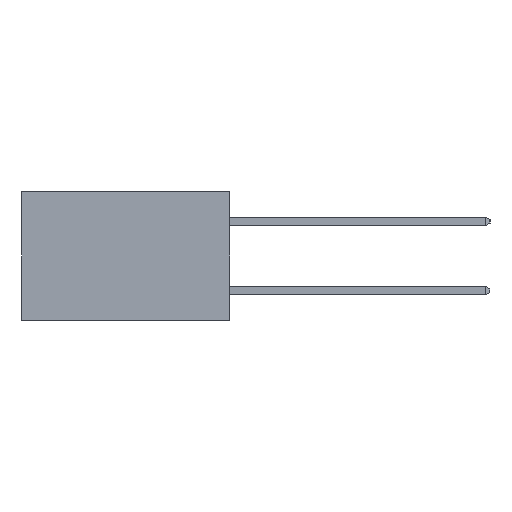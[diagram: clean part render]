
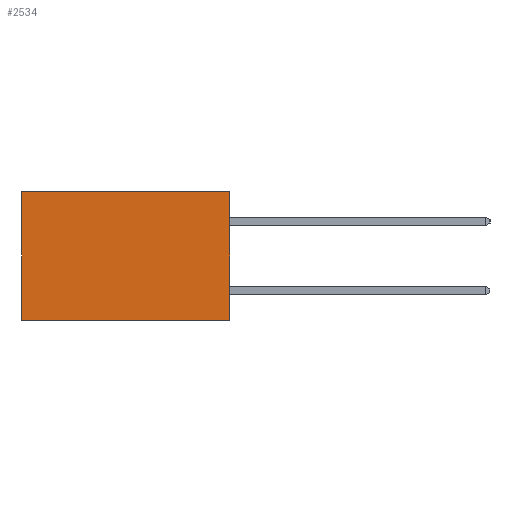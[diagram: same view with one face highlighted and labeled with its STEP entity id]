
A CAD part, left-side view. The second image highlights one B-rep face of the part: STEP entity #2534.
In plain terms, the highlighted planar face has unit normal (-1, 0, 0).
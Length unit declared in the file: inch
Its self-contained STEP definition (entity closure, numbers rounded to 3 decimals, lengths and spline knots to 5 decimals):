
#65 = DIRECTION ( 'NONE',  ( 1., 0., 0. ) ) ;
#964 = LINE ( 'NONE', #3875, #15997 ) ;
#1285 = CARTESIAN_POINT ( 'NONE',  ( 0.298, 0., 0. ) ) ;
#1980 = EDGE_CURVE ( 'NONE', #6765, #12540, #15928, .T. ) ;
#2534 = ADVANCED_FACE ( 'NONE', ( #10368 ), #13266, .F. ) ;
#2613 = VECTOR ( 'NONE', #5511, 39.37008 ) ;
#2827 = DIRECTION ( 'NONE',  ( 0., 1., 0. ) ) ;
#3875 = CARTESIAN_POINT ( 'NONE',  ( 0.298, 0.6, 0. ) ) ;
#4779 = EDGE_CURVE ( 'NONE', #13576, #14364, #964, .T. ) ;
#5061 = CARTESIAN_POINT ( 'NONE',  ( 0.298, 0., -0.37 ) ) ;
#5412 = CARTESIAN_POINT ( 'NONE',  ( 0.298, 0., 0. ) ) ;
#5511 = DIRECTION ( 'NONE',  ( 0., 1., 0. ) ) ;
#6765 = VERTEX_POINT ( 'NONE', #5412 ) ;
#7298 = CARTESIAN_POINT ( 'NONE',  ( 0.298, 0.6, 0. ) ) ;
#8626 = LINE ( 'NONE', #18253, #2613 ) ;
#9124 = EDGE_CURVE ( 'NONE', #6765, #13576, #18658, .T. ) ;
#9992 = ORIENTED_EDGE ( 'NONE', *, *, #9124, .T. ) ;
#10171 = ORIENTED_EDGE ( 'NONE', *, *, #4779, .T. ) ;
#10368 = FACE_OUTER_BOUND ( 'NONE', #14042, .T. ) ;
#10563 = ORIENTED_EDGE ( 'NONE', *, *, #1980, .F. ) ;
#11059 = EDGE_CURVE ( 'NONE', #12540, #14364, #8626, .T. ) ;
#11389 = CARTESIAN_POINT ( 'NONE',  ( 0.298, 0., 0. ) ) ;
#11412 = DIRECTION ( 'NONE',  ( 0., 0., -1. ) ) ;
#11828 = ORIENTED_EDGE ( 'NONE', *, *, #11059, .F. ) ;
#12179 = VECTOR ( 'NONE', #11412, 39.37008 ) ;
#12540 = VERTEX_POINT ( 'NONE', #5061 ) ;
#12905 = DIRECTION ( 'NONE',  ( 0., 0., -1. ) ) ;
#13076 = DIRECTION ( 'NONE',  ( 0., 0., -1. ) ) ;
#13266 = PLANE ( 'NONE',  #15378 ) ;
#13347 = CARTESIAN_POINT ( 'NONE',  ( 0.298, 0., 0. ) ) ;
#13576 = VERTEX_POINT ( 'NONE', #7298 ) ;
#14042 = EDGE_LOOP ( 'NONE', ( #10171, #11828, #10563, #9992 ) ) ;
#14364 = VERTEX_POINT ( 'NONE', #14714 ) ;
#14714 = CARTESIAN_POINT ( 'NONE',  ( 0.298, 0.6, -0.37 ) ) ;
#15378 = AXIS2_PLACEMENT_3D ( 'NONE', #13347, #65, #12905 ) ;
#15928 = LINE ( 'NONE', #11389, #12179 ) ;
#15997 = VECTOR ( 'NONE', #13076, 39.37008 ) ;
#18229 = VECTOR ( 'NONE', #2827, 39.37008 ) ;
#18253 = CARTESIAN_POINT ( 'NONE',  ( 0.298, 0., -0.37 ) ) ;
#18658 = LINE ( 'NONE', #1285, #18229 ) ;
